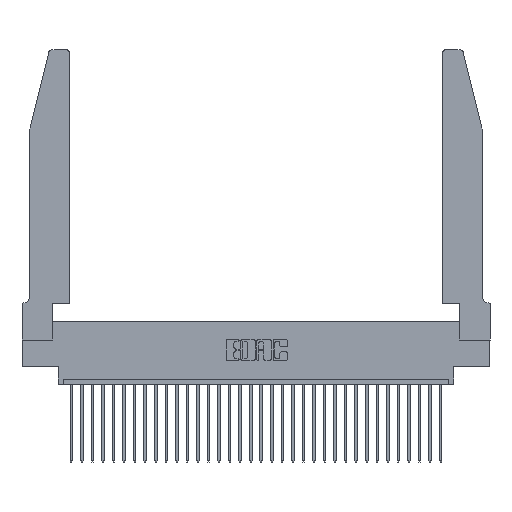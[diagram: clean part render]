
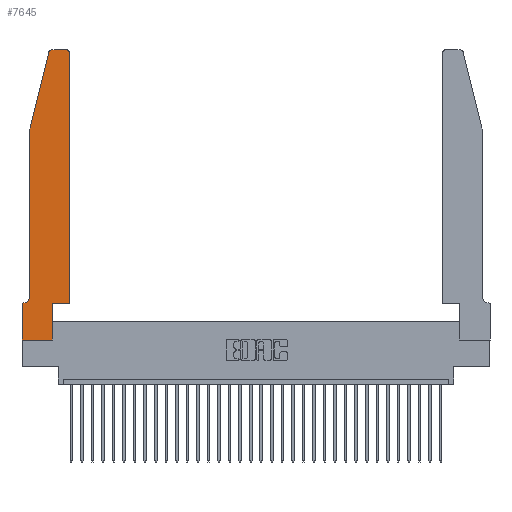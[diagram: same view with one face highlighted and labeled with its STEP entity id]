
A CAD part, top view. The second image highlights one B-rep face of the part: STEP entity #7645.
In plain terms, the highlighted planar face has unit normal (0, 0, 1).
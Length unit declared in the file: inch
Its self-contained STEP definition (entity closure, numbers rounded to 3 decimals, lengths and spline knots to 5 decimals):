
#7 = EDGE_CURVE ( 'NONE', #2665, #15693, #27479, .T. ) ;
#143 = VERTEX_POINT ( 'NONE', #5755 ) ;
#381 = VERTEX_POINT ( 'NONE', #27881 ) ;
#1263 = VECTOR ( 'NONE', #12398, 39.37008 ) ;
#1748 = DIRECTION ( 'NONE',  ( 0., 0., 1. ) ) ;
#1751 = VERTEX_POINT ( 'NONE', #27050 ) ;
#1888 = CARTESIAN_POINT ( 'NONE',  ( 0.0755, 2., 0.37 ) ) ;
#2665 = VERTEX_POINT ( 'NONE', #11150 ) ;
#3048 = ORIENTED_EDGE ( 'NONE', *, *, #11044, .T. ) ;
#3483 = AXIS2_PLACEMENT_3D ( 'NONE', #30310, #20381, #15217 ) ;
#4664 = CIRCLE ( 'NONE', #7516, 0.03 ) ;
#4719 = VERTEX_POINT ( 'NONE', #15225 ) ;
#4762 = CARTESIAN_POINT ( 'NONE',  ( 0.284, 2.72, 0.37 ) ) ;
#5027 = LINE ( 'NONE', #27061, #14605 ) ;
#5404 = ORIENTED_EDGE ( 'NONE', *, *, #8177, .T. ) ;
#5407 = DIRECTION ( 'NONE',  ( -1., 0., 0. ) ) ;
#5755 = CARTESIAN_POINT ( 'NONE',  ( 0.25487, 2.72718, 0.37 ) ) ;
#5936 = ORIENTED_EDGE ( 'NONE', *, *, #7, .T. ) ;
#6802 = CARTESIAN_POINT ( 'NONE',  ( 0.0755, 0.42, 0.37 ) ) ;
#6993 = CIRCLE ( 'NONE', #31228, 0.07 ) ;
#7078 = DIRECTION ( 'NONE',  ( 0., 1., 0. ) ) ;
#7188 = EDGE_CURVE ( 'NONE', #15693, #143, #4664, .T. ) ;
#7274 = DIRECTION ( 'NONE',  ( 1., 0., 0. ) ) ;
#7475 = PLANE ( 'NONE',  #24944 ) ;
#7516 = AXIS2_PLACEMENT_3D ( 'NONE', #4762, #1748, #12246 ) ;
#7645 = ADVANCED_FACE ( 'NONE', ( #30733 ), #7475, .T. ) ;
#7948 = VECTOR ( 'NONE', #12468, 39.37008 ) ;
#8172 = DIRECTION ( 'NONE',  ( -0.239, -0.971, 0. ) ) ;
#8177 = EDGE_CURVE ( 'NONE', #16907, #24608, #6993, .T. ) ;
#8412 = ORIENTED_EDGE ( 'NONE', *, *, #9243, .T. ) ;
#8651 = VECTOR ( 'NONE', #32801, 39.37008 ) ;
#9102 = LINE ( 'NONE', #27105, #13843 ) ;
#9235 = ORIENTED_EDGE ( 'NONE', *, *, #22708, .T. ) ;
#9243 = EDGE_CURVE ( 'NONE', #143, #381, #18403, .T. ) ;
#9340 = VERTEX_POINT ( 'NONE', #22106 ) ;
#9949 = DIRECTION ( 'NONE',  ( 0., 0., 1. ) ) ;
#10147 = CARTESIAN_POINT ( 'NONE',  ( 0., 0.35, 0.37 ) ) ;
#10172 = VECTOR ( 'NONE', #24332, 39.37008 ) ;
#10224 = CARTESIAN_POINT ( 'NONE',  ( 0.0055, 0.35, 0.37 ) ) ;
#10455 = VECTOR ( 'NONE', #8172, 39.37008 ) ;
#10927 = ORIENTED_EDGE ( 'NONE', *, *, #30660, .T. ) ;
#11044 = EDGE_CURVE ( 'NONE', #381, #16907, #21842, .T. ) ;
#11150 = CARTESIAN_POINT ( 'NONE',  ( 0.4205, 2.75, 0.37 ) ) ;
#12184 = EDGE_LOOP ( 'NONE', ( #5936, #28413, #8412, #3048, #5404, #18638, #9235, #10927, #27628, #28909, #12309, #21284 ) ) ;
#12246 = DIRECTION ( 'NONE',  ( 1., 0., 0. ) ) ;
#12309 = ORIENTED_EDGE ( 'NONE', *, *, #19249, .T. ) ;
#12398 = DIRECTION ( 'NONE',  ( -1., 0., 0. ) ) ;
#12468 = DIRECTION ( 'NONE',  ( 0., -1., 0. ) ) ;
#12473 = VERTEX_POINT ( 'NONE', #20259 ) ;
#12986 = CIRCLE ( 'NONE', #3483, 0.03 ) ;
#13008 = CARTESIAN_POINT ( 'NONE',  ( 0.0055, 0.42, 0.37 ) ) ;
#13635 = VECTOR ( 'NONE', #23868, 39.37008 ) ;
#13713 = LINE ( 'NONE', #31682, #16086 ) ;
#13843 = VECTOR ( 'NONE', #7078, 39.37008 ) ;
#14605 = VECTOR ( 'NONE', #24967, 39.37008 ) ;
#15157 = CARTESIAN_POINT ( 'NONE',  ( 0., 0., 0.37 ) ) ;
#15217 = DIRECTION ( 'NONE',  ( 1., 0., 0. ) ) ;
#15225 = CARTESIAN_POINT ( 'NONE',  ( 0.4505, 2.72, 0.37 ) ) ;
#15253 = LINE ( 'NONE', #31353, #13635 ) ;
#15693 = VERTEX_POINT ( 'NONE', #19503 ) ;
#16086 = VECTOR ( 'NONE', #19143, 39.37008 ) ;
#16900 = LINE ( 'NONE', #19053, #10172 ) ;
#16907 = VERTEX_POINT ( 'NONE', #6802 ) ;
#17096 = CARTESIAN_POINT ( 'NONE',  ( 0.2865, 0., 0.37 ) ) ;
#18403 = LINE ( 'NONE', #28310, #10455 ) ;
#18638 = ORIENTED_EDGE ( 'NONE', *, *, #29595, .T. ) ;
#19053 = CARTESIAN_POINT ( 'NONE',  ( 0., 0., 0.37 ) ) ;
#19143 = DIRECTION ( 'NONE',  ( 1., 0., 0. ) ) ;
#19249 = EDGE_CURVE ( 'NONE', #12473, #4719, #15253, .T. ) ;
#19503 = CARTESIAN_POINT ( 'NONE',  ( 0.284, 2.75, 0.37 ) ) ;
#20259 = CARTESIAN_POINT ( 'NONE',  ( 0.4505, 0.35, 0.37 ) ) ;
#20381 = DIRECTION ( 'NONE',  ( 0., 0., 1. ) ) ;
#20623 = DIRECTION ( 'NONE',  ( 0., 0., -1. ) ) ;
#21284 = ORIENTED_EDGE ( 'NONE', *, *, #23175, .T. ) ;
#21842 = LINE ( 'NONE', #1888, #7948 ) ;
#22106 = CARTESIAN_POINT ( 'NONE',  ( 0., 0., 0.37 ) ) ;
#22455 = CARTESIAN_POINT ( 'NONE',  ( 0.2605, 2.75, 0.37 ) ) ;
#22708 = EDGE_CURVE ( 'NONE', #1751, #9340, #30405, .T. ) ;
#23175 = EDGE_CURVE ( 'NONE', #4719, #2665, #12986, .T. ) ;
#23868 = DIRECTION ( 'NONE',  ( 0., 1., 0. ) ) ;
#24332 = DIRECTION ( 'NONE',  ( 1., 0., 0. ) ) ;
#24608 = VERTEX_POINT ( 'NONE', #10224 ) ;
#24944 = AXIS2_PLACEMENT_3D ( 'NONE', #10147, #9949, #7274 ) ;
#24967 = DIRECTION ( 'NONE',  ( -1., 0., 0. ) ) ;
#27050 = CARTESIAN_POINT ( 'NONE',  ( 0., 0.35, 0.37 ) ) ;
#27061 = CARTESIAN_POINT ( 'NONE',  ( 0.0755, 0.35, 0.37 ) ) ;
#27105 = CARTESIAN_POINT ( 'NONE',  ( 0.2865, 0.35, 0.37 ) ) ;
#27479 = LINE ( 'NONE', #22455, #1263 ) ;
#27628 = ORIENTED_EDGE ( 'NONE', *, *, #28899, .T. ) ;
#27677 = VERTEX_POINT ( 'NONE', #17096 ) ;
#27881 = CARTESIAN_POINT ( 'NONE',  ( 0.0755, 2., 0.37 ) ) ;
#28310 = CARTESIAN_POINT ( 'NONE',  ( 0.0755, 2., 0.37 ) ) ;
#28413 = ORIENTED_EDGE ( 'NONE', *, *, #7188, .T. ) ;
#28899 = EDGE_CURVE ( 'NONE', #27677, #29783, #9102, .T. ) ;
#28909 = ORIENTED_EDGE ( 'NONE', *, *, #31150, .T. ) ;
#29595 = EDGE_CURVE ( 'NONE', #24608, #1751, #5027, .T. ) ;
#29783 = VERTEX_POINT ( 'NONE', #30424 ) ;
#30310 = CARTESIAN_POINT ( 'NONE',  ( 0.4205, 2.72, 0.37 ) ) ;
#30405 = LINE ( 'NONE', #15157, #8651 ) ;
#30424 = CARTESIAN_POINT ( 'NONE',  ( 0.2865, 0.35, 0.37 ) ) ;
#30660 = EDGE_CURVE ( 'NONE', #9340, #27677, #16900, .T. ) ;
#30733 = FACE_OUTER_BOUND ( 'NONE', #12184, .T. ) ;
#31150 = EDGE_CURVE ( 'NONE', #29783, #12473, #13713, .T. ) ;
#31228 = AXIS2_PLACEMENT_3D ( 'NONE', #13008, #20623, #5407 ) ;
#31353 = CARTESIAN_POINT ( 'NONE',  ( 0.4505, 0.35, 0.37 ) ) ;
#31682 = CARTESIAN_POINT ( 'NONE',  ( 0.4505, 0.35, 0.37 ) ) ;
#32801 = DIRECTION ( 'NONE',  ( 0., -1., 0. ) ) ;
